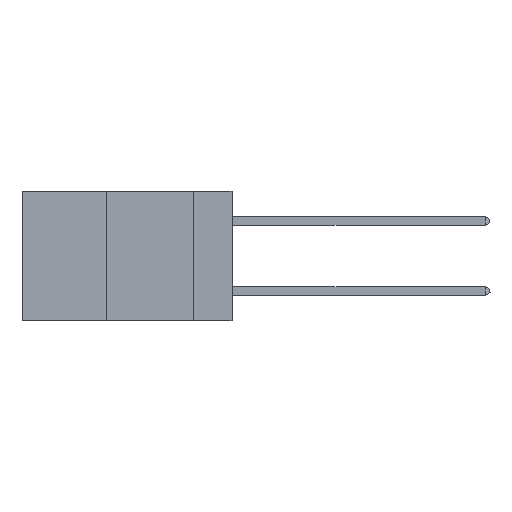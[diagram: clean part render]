
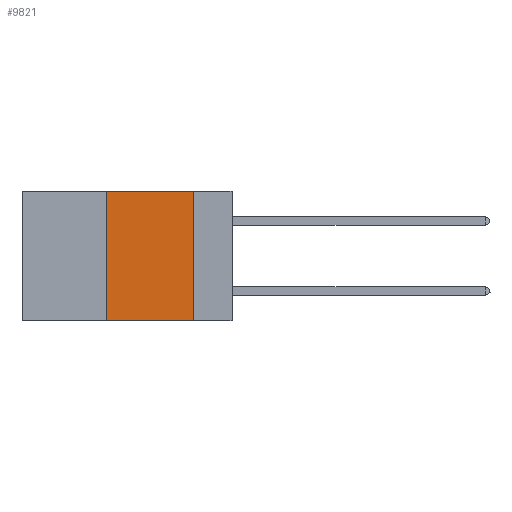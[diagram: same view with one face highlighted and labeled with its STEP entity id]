
A CAD part, left-side view. The second image highlights one B-rep face of the part: STEP entity #9821.
In plain terms, the highlighted planar face has unit normal (-1, 0, 0).
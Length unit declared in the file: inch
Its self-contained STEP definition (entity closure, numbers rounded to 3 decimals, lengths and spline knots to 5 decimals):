
#881 = VERTEX_POINT ( 'NONE', #20934 ) ;
#1819 = ORIENTED_EDGE ( 'NONE', *, *, #24008, .F. ) ;
#2345 = ORIENTED_EDGE ( 'NONE', *, *, #25515, .F. ) ;
#2599 = VERTEX_POINT ( 'NONE', #13139 ) ;
#4481 = ORIENTED_EDGE ( 'NONE', *, *, #16768, .F. ) ;
#4889 = EDGE_CURVE ( 'NONE', #6594, #881, #16789, .T. ) ;
#5841 = DIRECTION ( 'NONE',  ( 0., -1., 0. ) ) ;
#6594 = VERTEX_POINT ( 'NONE', #18659 ) ;
#7927 = DIRECTION ( 'NONE',  ( 0., 0., 1. ) ) ;
#9063 = EDGE_LOOP ( 'NONE', ( #1819, #4481, #2345, #13382 ) ) ;
#9337 = DIRECTION ( 'NONE',  ( 0., 0., -1. ) ) ;
#9821 = ADVANCED_FACE ( 'NONE', ( #24175 ), #28052, .F. ) ;
#11643 = DIRECTION ( 'NONE',  ( 1., 0., 0. ) ) ;
#13024 = CARTESIAN_POINT ( 'NONE',  ( 0., 0.6, 0. ) ) ;
#13139 = CARTESIAN_POINT ( 'NONE',  ( 0., 0.36, 0. ) ) ;
#13382 = ORIENTED_EDGE ( 'NONE', *, *, #4889, .T. ) ;
#14861 = DIRECTION ( 'NONE',  ( 0., -1., 0. ) ) ;
#14885 = VERTEX_POINT ( 'NONE', #15716 ) ;
#14905 = VECTOR ( 'NONE', #14861, 39.37008 ) ;
#15716 = CARTESIAN_POINT ( 'NONE',  ( 0., 0.11, 0. ) ) ;
#15833 = CARTESIAN_POINT ( 'NONE',  ( 0., 0.6, -0.37 ) ) ;
#16768 = EDGE_CURVE ( 'NONE', #2599, #14885, #29297, .T. ) ;
#16789 = LINE ( 'NONE', #15833, #14905 ) ;
#17432 = CARTESIAN_POINT ( 'NONE',  ( 0., 0.36, 0. ) ) ;
#18659 = CARTESIAN_POINT ( 'NONE',  ( 0., 0.36, -0.37 ) ) ;
#20934 = CARTESIAN_POINT ( 'NONE',  ( 0., 0.11, -0.37 ) ) ;
#21029 = DIRECTION ( 'NONE',  ( 0., 0., -1. ) ) ;
#21871 = LINE ( 'NONE', #23228, #23371 ) ;
#22322 = VECTOR ( 'NONE', #7927, 39.37008 ) ;
#23228 = CARTESIAN_POINT ( 'NONE',  ( 0., 0.11, 0. ) ) ;
#23371 = VECTOR ( 'NONE', #21029, 39.37008 ) ;
#23620 = CARTESIAN_POINT ( 'NONE',  ( 0., 0.6, 0. ) ) ;
#24008 = EDGE_CURVE ( 'NONE', #14885, #881, #21871, .T. ) ;
#24175 = FACE_OUTER_BOUND ( 'NONE', #9063, .T. ) ;
#25515 = EDGE_CURVE ( 'NONE', #6594, #2599, #29058, .T. ) ;
#28052 = PLANE ( 'NONE',  #30227 ) ;
#29058 = LINE ( 'NONE', #17432, #22322 ) ;
#29297 = LINE ( 'NONE', #13024, #30770 ) ;
#30227 = AXIS2_PLACEMENT_3D ( 'NONE', #23620, #11643, #9337 ) ;
#30770 = VECTOR ( 'NONE', #5841, 39.37008 ) ;
